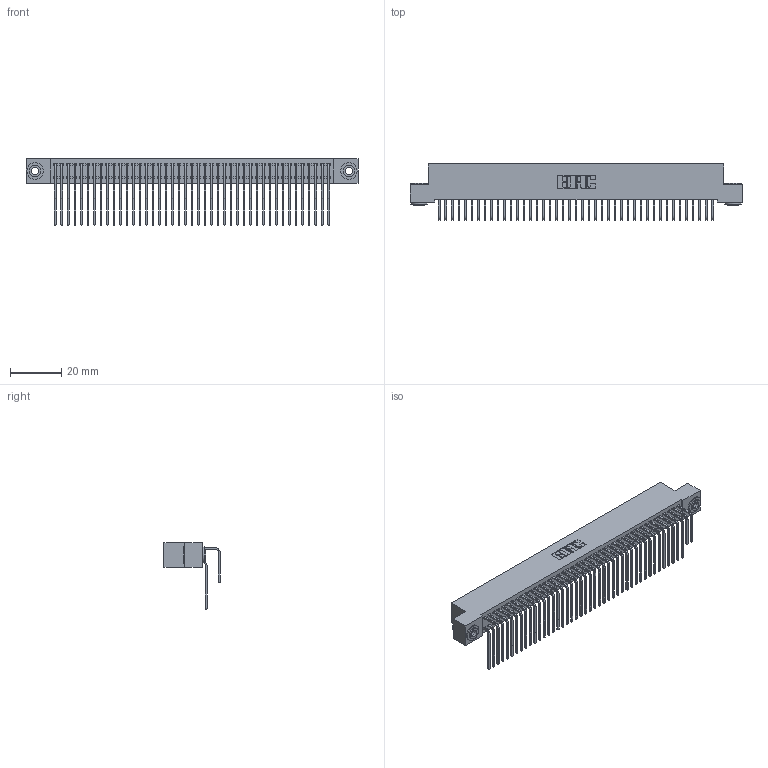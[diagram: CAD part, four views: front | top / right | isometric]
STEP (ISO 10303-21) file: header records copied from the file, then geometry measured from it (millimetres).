
FILE_DESCRIPTION (( 'STEP AP203' ), '1' );
FILE_NAME ('392-086-558-203.STEP', '2018-08-18T05:39:01', ( '' ), ( '' ), 'SwSTEP 2.0', 'SolidWorks 2016', '' );
FILE_SCHEMA (( 'CONFIG_CONTROL_DESIGN' ));
Length unit declared in the file: inch
Products named in the file (5): 342-250-002_345-250-002-102; 392-086-558-203; 342 Part_.156 TH; 345-292-001_558 559 Tail - 1; 345-292-001_558 Tail - 2
Assembly tree (89 placements, depth 2):
  392-086-558-203
    342 Part_.156 TH
    345-292-001_558 559 Tail - 1  x43
    345-292-001_558 Tail - 2  x43
    342-250-002_345-250-002-102  x2
Bounding box: 129.54 x 21.91 x 25.78 mm (x, y, z)
Volume: 12162.8 mm3; surface area: 22281 mm2
Topology: 89 solids, 89 shells, 4792 faces, 14221 edges, 9362 vertices
Faces by surface type: plane 3344, cylinder 1440, cone 8
Entity records: 29836 total; most frequent: CARTESIAN_POINT 4968, ORIENTED_EDGE 4846, DIRECTION 4257, EDGE_CURVE 2423, LINE 2231, VECTOR 2231, VERTEX_POINT 1610, AXIS2_PLACEMENT_3D 1013
